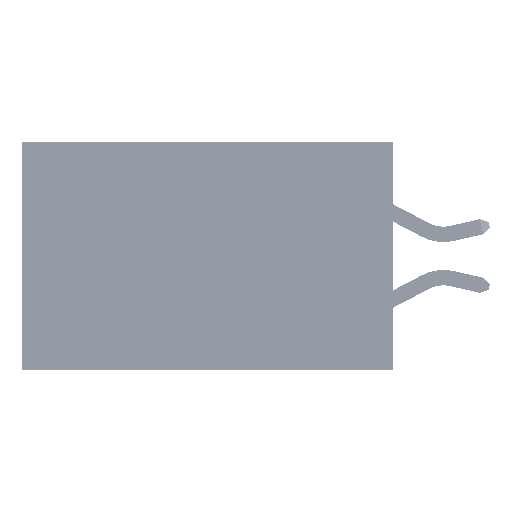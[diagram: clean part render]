
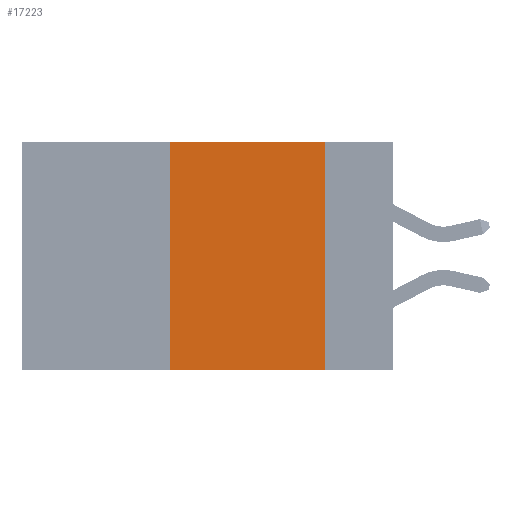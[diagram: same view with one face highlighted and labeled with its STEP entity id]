
A CAD part, left-side view. The second image highlights one B-rep face of the part: STEP entity #17223.
In plain terms, the highlighted planar face has unit normal (-1, 0, 0).
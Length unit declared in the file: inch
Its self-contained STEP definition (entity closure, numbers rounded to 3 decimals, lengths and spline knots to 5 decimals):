
#22 = CARTESIAN_POINT ( 'NONE',  ( 0., 0.6, 0. ) ) ;
#1806 = DIRECTION ( 'NONE',  ( 0., 0., -1. ) ) ;
#2499 = DIRECTION ( 'NONE',  ( 0., 0., 1. ) ) ;
#2772 = DIRECTION ( 'NONE',  ( 0., -1., 0. ) ) ;
#3021 = ORIENTED_EDGE ( 'NONE', *, *, #12861, .F. ) ;
#3092 = VECTOR ( 'NONE', #2772, 39.37008 ) ;
#4403 = AXIS2_PLACEMENT_3D ( 'NONE', #22, #37490, #18462 ) ;
#4597 = FACE_OUTER_BOUND ( 'NONE', #20688, .T. ) ;
#9169 = CARTESIAN_POINT ( 'NONE',  ( 0., 0.36, -0.37 ) ) ;
#10896 = PLANE ( 'NONE',  #4403 ) ;
#10931 = VERTEX_POINT ( 'NONE', #29235 ) ;
#12861 = EDGE_CURVE ( 'NONE', #10931, #15839, #36358, .T. ) ;
#14086 = VERTEX_POINT ( 'NONE', #9169 ) ;
#14160 = CARTESIAN_POINT ( 'NONE',  ( 0., 0.36, 0. ) ) ;
#15839 = VERTEX_POINT ( 'NONE', #30856 ) ;
#17223 = ADVANCED_FACE ( 'NONE', ( #4597 ), #10896, .F. ) ;
#18462 = DIRECTION ( 'NONE',  ( 0., 0., -1. ) ) ;
#18970 = LINE ( 'NONE', #27982, #43878 ) ;
#19943 = CARTESIAN_POINT ( 'NONE',  ( 0., 0.11, -0.37 ) ) ;
#20688 = EDGE_LOOP ( 'NONE', ( #36607, #3021, #35506, #45070 ) ) ;
#21942 = CARTESIAN_POINT ( 'NONE',  ( 0., 0.6, 0. ) ) ;
#22158 = CARTESIAN_POINT ( 'NONE',  ( 0., 0.6, -0.37 ) ) ;
#24649 = EDGE_CURVE ( 'NONE', #14086, #10931, #38589, .T. ) ;
#25049 = EDGE_CURVE ( 'NONE', #15839, #40274, #18970, .T. ) ;
#26650 = LINE ( 'NONE', #22158, #3092 ) ;
#27982 = CARTESIAN_POINT ( 'NONE',  ( 0., 0.11, 0. ) ) ;
#29235 = CARTESIAN_POINT ( 'NONE',  ( 0., 0.36, 0. ) ) ;
#30856 = CARTESIAN_POINT ( 'NONE',  ( 0., 0.11, 0. ) ) ;
#31145 = EDGE_CURVE ( 'NONE', #14086, #40274, #26650, .T. ) ;
#32175 = VECTOR ( 'NONE', #44511, 39.37008 ) ;
#35506 = ORIENTED_EDGE ( 'NONE', *, *, #24649, .F. ) ;
#36358 = LINE ( 'NONE', #21942, #32175 ) ;
#36607 = ORIENTED_EDGE ( 'NONE', *, *, #25049, .F. ) ;
#37389 = VECTOR ( 'NONE', #2499, 39.37008 ) ;
#37490 = DIRECTION ( 'NONE',  ( 1., 0., 0. ) ) ;
#38589 = LINE ( 'NONE', #14160, #37389 ) ;
#40274 = VERTEX_POINT ( 'NONE', #19943 ) ;
#43878 = VECTOR ( 'NONE', #1806, 39.37008 ) ;
#44511 = DIRECTION ( 'NONE',  ( 0., -1., 0. ) ) ;
#45070 = ORIENTED_EDGE ( 'NONE', *, *, #31145, .T. ) ;
